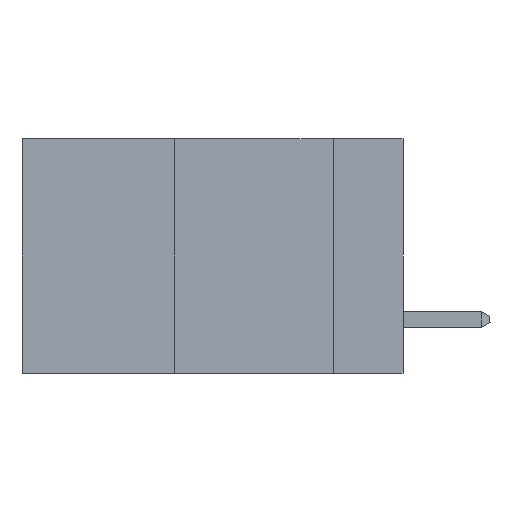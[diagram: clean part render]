
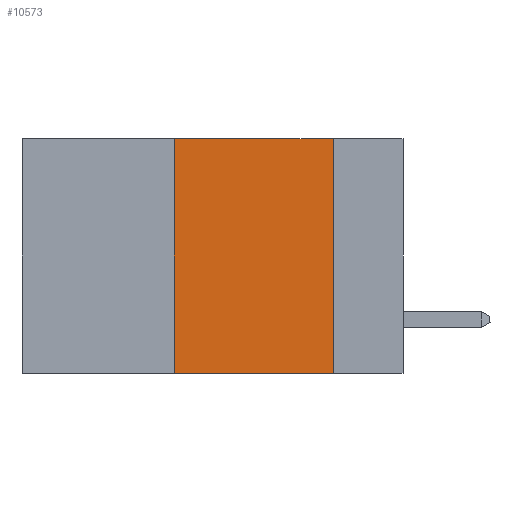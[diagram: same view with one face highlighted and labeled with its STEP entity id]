
A CAD part, left-side view. The second image highlights one B-rep face of the part: STEP entity #10573.
In plain terms, the highlighted planar face has unit normal (-1, 0, 0).
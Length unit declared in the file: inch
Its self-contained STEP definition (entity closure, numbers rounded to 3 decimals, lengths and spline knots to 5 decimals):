
#902 = EDGE_CURVE ( 'NONE', #5667, #13645, #9913, .T. ) ;
#1641 = DIRECTION ( 'NONE',  ( 0., -1., 0. ) ) ;
#2267 = CARTESIAN_POINT ( 'NONE',  ( 0., 0.11, -0.37 ) ) ;
#2660 = ORIENTED_EDGE ( 'NONE', *, *, #7233, .F. ) ;
#3092 = CARTESIAN_POINT ( 'NONE',  ( 0., 0.36, 0. ) ) ;
#3530 = EDGE_LOOP ( 'NONE', ( #17292, #3649, #2660, #8505 ) ) ;
#3649 = ORIENTED_EDGE ( 'NONE', *, *, #16381, .F. ) ;
#4092 = CARTESIAN_POINT ( 'NONE',  ( 0., 0.6, -0.37 ) ) ;
#4344 = VECTOR ( 'NONE', #1641, 39.37008 ) ;
#4530 = VECTOR ( 'NONE', #19466, 39.37008 ) ;
#4969 = LINE ( 'NONE', #3092, #10323 ) ;
#5584 = CARTESIAN_POINT ( 'NONE',  ( 0., 0.11, 0. ) ) ;
#5667 = VERTEX_POINT ( 'NONE', #5584 ) ;
#6399 = EDGE_CURVE ( 'NONE', #6532, #13645, #13504, .T. ) ;
#6532 = VERTEX_POINT ( 'NONE', #19119 ) ;
#7233 = EDGE_CURVE ( 'NONE', #6532, #13420, #4969, .T. ) ;
#7896 = DIRECTION ( 'NONE',  ( 0., 0., 1. ) ) ;
#7964 = VECTOR ( 'NONE', #17831, 39.37008 ) ;
#8505 = ORIENTED_EDGE ( 'NONE', *, *, #6399, .T. ) ;
#9913 = LINE ( 'NONE', #16458, #7964 ) ;
#10323 = VECTOR ( 'NONE', #7896, 39.37008 ) ;
#10418 = CARTESIAN_POINT ( 'NONE',  ( 0., 0.36, 0. ) ) ;
#10573 = ADVANCED_FACE ( 'NONE', ( #15728 ), #11567, .F. ) ;
#11567 = PLANE ( 'NONE',  #18994 ) ;
#13253 = DIRECTION ( 'NONE',  ( 1., 0., 0. ) ) ;
#13420 = VERTEX_POINT ( 'NONE', #10418 ) ;
#13504 = LINE ( 'NONE', #4092, #4530 ) ;
#13645 = VERTEX_POINT ( 'NONE', #2267 ) ;
#15681 = CARTESIAN_POINT ( 'NONE',  ( 0., 0.6, 0. ) ) ;
#15728 = FACE_OUTER_BOUND ( 'NONE', #3530, .T. ) ;
#16381 = EDGE_CURVE ( 'NONE', #13420, #5667, #19320, .T. ) ;
#16458 = CARTESIAN_POINT ( 'NONE',  ( 0., 0.11, 0. ) ) ;
#17292 = ORIENTED_EDGE ( 'NONE', *, *, #902, .F. ) ;
#17796 = DIRECTION ( 'NONE',  ( 0., 0., -1. ) ) ;
#17831 = DIRECTION ( 'NONE',  ( 0., 0., -1. ) ) ;
#18994 = AXIS2_PLACEMENT_3D ( 'NONE', #19335, #13253, #17796 ) ;
#19119 = CARTESIAN_POINT ( 'NONE',  ( 0., 0.36, -0.37 ) ) ;
#19320 = LINE ( 'NONE', #15681, #4344 ) ;
#19335 = CARTESIAN_POINT ( 'NONE',  ( 0., 0.6, 0. ) ) ;
#19466 = DIRECTION ( 'NONE',  ( 0., -1., 0. ) ) ;
